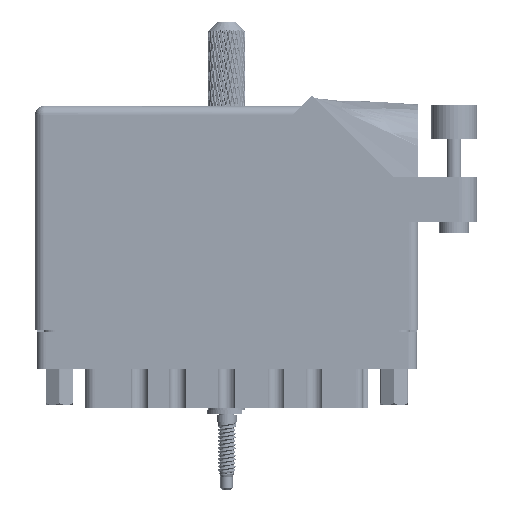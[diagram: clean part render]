
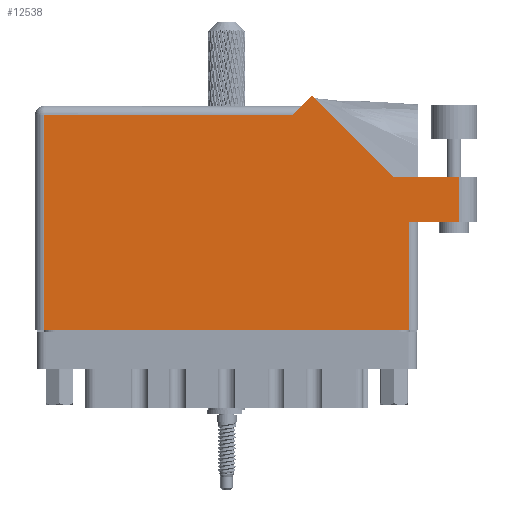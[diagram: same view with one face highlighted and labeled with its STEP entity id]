
A CAD part, front view. The second image highlights one B-rep face of the part: STEP entity #12538.
In plain terms, the highlighted face is planar.
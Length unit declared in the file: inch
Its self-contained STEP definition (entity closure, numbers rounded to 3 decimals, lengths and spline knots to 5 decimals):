
#830 = VERTEX_POINT ( 'NONE', #16883 ) ;
#1534 = EDGE_CURVE ( 'NONE', #63438, #64007, #72368, .T. ) ;
#1849 = EDGE_CURVE ( 'NONE', #79361, #117261, #31400, .T. ) ;
#2182 = PLANE ( 'NONE',  #94601 ) ;
#3285 = VECTOR ( 'NONE', #72071, 39.37008 ) ;
#7282 = VECTOR ( 'NONE', #18229, 39.37008 ) ;
#9237 = VERTEX_POINT ( 'NONE', #77857 ) ;
#10628 = EDGE_CURVE ( 'NONE', #9237, #830, #12665, .T. ) ;
#11939 = CARTESIAN_POINT ( 'NONE',  ( 0., 0., 0. ) ) ;
#12538 = ADVANCED_FACE ( 'NONE', ( #89050 ), #2182, .F. ) ;
#12665 = LINE ( 'NONE', #13952, #101758 ) ;
#13952 = CARTESIAN_POINT ( 'NONE',  ( 1.819, 1.53, 0. ) ) ;
#15943 = LINE ( 'NONE', #114420, #94743 ) ;
#16583 = DIRECTION ( 'NONE',  ( -1., 0., 0. ) ) ;
#16883 = CARTESIAN_POINT ( 'NONE',  ( 1.757, 1.468, 0. ) ) ;
#18229 = DIRECTION ( 'NONE',  ( 1., 0., 0. ) ) ;
#19442 = ORIENTED_EDGE ( 'NONE', *, *, #78370, .T. ) ;
#20579 = ORIENTED_EDGE ( 'NONE', *, *, #44743, .T. ) ;
#21043 = DIRECTION ( 'NONE',  ( 1., 0., 0. ) ) ;
#21477 = CARTESIAN_POINT ( 'NONE',  ( 2.55, 0., 0. ) ) ;
#21505 = EDGE_LOOP ( 'NONE', ( #37763, #70755, #61406, #99273, #29139, #109503, #19442, #86396, #20579 ) ) ;
#25414 = VECTOR ( 'NONE', #66072, 39.37008 ) ;
#29139 = ORIENTED_EDGE ( 'NONE', *, *, #10628, .T. ) ;
#31400 = LINE ( 'NONE', #11939, #65171 ) ;
#31546 = LINE ( 'NONE', #40668, #80029 ) ;
#32416 = CARTESIAN_POINT ( 'NONE',  ( 3.012, 1.044, 0. ) ) ;
#35428 = CARTESIAN_POINT ( 'NONE',  ( 2.44642, 1.044, 0. ) ) ;
#37763 = ORIENTED_EDGE ( 'NONE', *, *, #50048, .T. ) ;
#40668 = CARTESIAN_POINT ( 'NONE',  ( 2.55, 0.737, 0. ) ) ;
#41531 = DIRECTION ( 'NONE',  ( -1., 0., 0. ) ) ;
#41637 = CARTESIAN_POINT ( 'NONE',  ( 2.44642, 1.044, 0. ) ) ;
#43152 = VECTOR ( 'NONE', #41531, 39.37008 ) ;
#44743 = EDGE_CURVE ( 'NONE', #117261, #87643, #31546, .T. ) ;
#47276 = CARTESIAN_POINT ( 'NONE',  ( 0.062, 0., 0. ) ) ;
#50048 = EDGE_CURVE ( 'NONE', #87643, #63438, #66877, .T. ) ;
#52770 = VECTOR ( 'NONE', #82718, 39.37008 ) ;
#61406 = ORIENTED_EDGE ( 'NONE', *, *, #108468, .T. ) ;
#63438 = VERTEX_POINT ( 'NONE', #93414 ) ;
#64007 = VERTEX_POINT ( 'NONE', #119112 ) ;
#65171 = VECTOR ( 'NONE', #21043, 39.37008 ) ;
#66072 = DIRECTION ( 'NONE',  ( 0., -1., 0. ) ) ;
#66877 = LINE ( 'NONE', #108888, #7282 ) ;
#68560 = VERTEX_POINT ( 'NONE', #110326 ) ;
#70755 = ORIENTED_EDGE ( 'NONE', *, *, #1534, .T. ) ;
#72071 = DIRECTION ( 'NONE',  ( -0.707, 0.707, 0. ) ) ;
#72368 = LINE ( 'NONE', #101499, #52770 ) ;
#73610 = VERTEX_POINT ( 'NONE', #35428 ) ;
#74219 = DIRECTION ( 'NONE',  ( -0.707, -0.707, 0. ) ) ;
#77857 = CARTESIAN_POINT ( 'NONE',  ( 1.88971, 1.60071, 0. ) ) ;
#78370 = EDGE_CURVE ( 'NONE', #68560, #79361, #114617, .T. ) ;
#79361 = VERTEX_POINT ( 'NONE', #92159 ) ;
#80029 = VECTOR ( 'NONE', #80807, 39.37008 ) ;
#80807 = DIRECTION ( 'NONE',  ( 0., 1., 0. ) ) ;
#81675 = LINE ( 'NONE', #32416, #43152 ) ;
#82718 = DIRECTION ( 'NONE',  ( 0., 1., 0. ) ) ;
#83047 = CARTESIAN_POINT ( 'NONE',  ( 2.55, 0.737, 0. ) ) ;
#86396 = ORIENTED_EDGE ( 'NONE', *, *, #1849, .T. ) ;
#87584 = EDGE_CURVE ( 'NONE', #73610, #9237, #109624, .T. ) ;
#87643 = VERTEX_POINT ( 'NONE', #83047 ) ;
#89050 = FACE_OUTER_BOUND ( 'NONE', #21505, .T. ) ;
#92159 = CARTESIAN_POINT ( 'NONE',  ( 0.062, 0., 0. ) ) ;
#93414 = CARTESIAN_POINT ( 'NONE',  ( 2.887, 0.737, 0. ) ) ;
#94601 = AXIS2_PLACEMENT_3D ( 'NONE', #98743, #99394, #119482 ) ;
#94743 = VECTOR ( 'NONE', #16583, 39.37008 ) ;
#95005 = EDGE_CURVE ( 'NONE', #830, #68560, #15943, .T. ) ;
#98743 = CARTESIAN_POINT ( 'NONE',  ( 0., 1.53, 0. ) ) ;
#99273 = ORIENTED_EDGE ( 'NONE', *, *, #87584, .T. ) ;
#99394 = DIRECTION ( 'NONE',  ( 0., 0., -1. ) ) ;
#101499 = CARTESIAN_POINT ( 'NONE',  ( 2.887, 1.044, 0. ) ) ;
#101758 = VECTOR ( 'NONE', #74219, 39.37008 ) ;
#108468 = EDGE_CURVE ( 'NONE', #64007, #73610, #81675, .T. ) ;
#108888 = CARTESIAN_POINT ( 'NONE',  ( 2.612, 0.737, 0. ) ) ;
#109503 = ORIENTED_EDGE ( 'NONE', *, *, #95005, .T. ) ;
#109624 = LINE ( 'NONE', #41637, #3285 ) ;
#110326 = CARTESIAN_POINT ( 'NONE',  ( 0.062, 1.468, 0. ) ) ;
#114420 = CARTESIAN_POINT ( 'NONE',  ( 0., 1.468, 0. ) ) ;
#114617 = LINE ( 'NONE', #47276, #25414 ) ;
#117261 = VERTEX_POINT ( 'NONE', #21477 ) ;
#119112 = CARTESIAN_POINT ( 'NONE',  ( 2.887, 1.044, 0. ) ) ;
#119482 = DIRECTION ( 'NONE',  ( -1., 0., 0. ) ) ;
